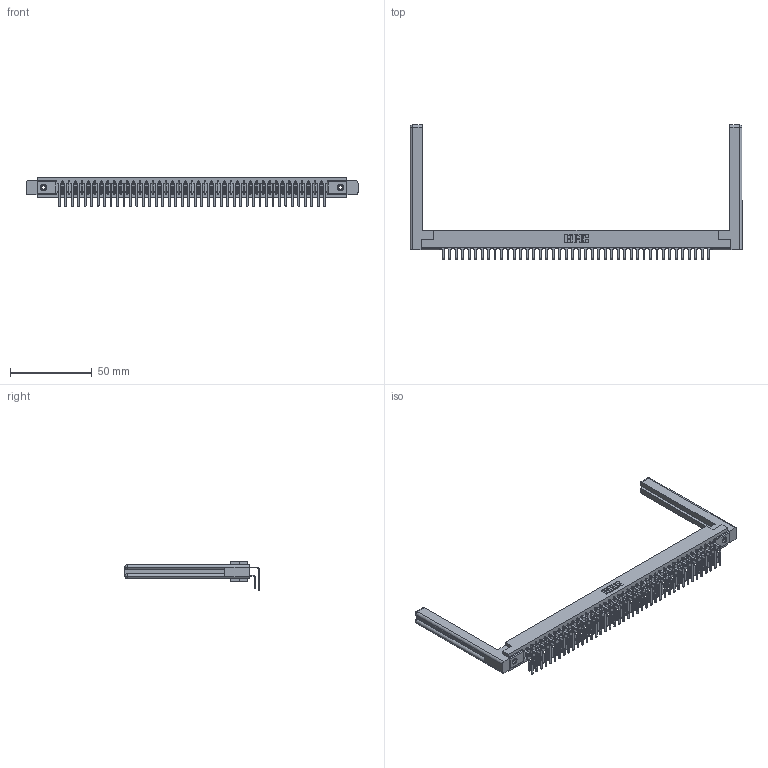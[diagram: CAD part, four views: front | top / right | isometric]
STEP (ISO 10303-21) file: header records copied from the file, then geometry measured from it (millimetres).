
FILE_DESCRIPTION (( 'STEP AP203' ), '1' );
FILE_NAME ('307-042-459-158.STEP', '2020-09-29T17:37:07', ( '' ), ( '' ), 'SwSTEP 2.0', 'SolidWorks 2020', '' );
FILE_SCHEMA (( 'CONFIG_CONTROL_DESIGN' ));
Length unit declared in the file: inch
Products named in the file (6): 307-220-058; 307-290-001_559 - 2 (Single); 307 Part_.156 Dia Mounting Holes; 307-290-001_558 559 - 1 (Single); 307-042-459-158; 345-250-001_345-250-001-102
Assembly tree (89 placements, depth 2):
  307-042-459-158
    307 Part_.156 Dia Mounting Holes
    307-290-001_558 559 - 1 (Single)  x42
    307-290-001_559 - 2 (Single)  x42
    307-220-058  x2
    345-250-001_345-250-001-102  x2
Bounding box: 203.05 x 82 x 18.07 mm (x, y, z)
Volume: 29093.5 mm3; surface area: 33937.2 mm2
Topology: 89 solids, 89 shells, 4503 faces, 12605 edges, 8162 vertices
Faces by surface type: plane 2926, cylinder 1467, sphere 86, torus 12, cone 12
Entity records: 41430 total; most frequent: CARTESIAN_POINT 6799, ORIENTED_EDGE 6680, DIRECTION 6616, EDGE_CURVE 3340, LINE 2558, VECTOR 2558, VERTEX_POINT 2158, AXIS2_PLACEMENT_3D 2029
